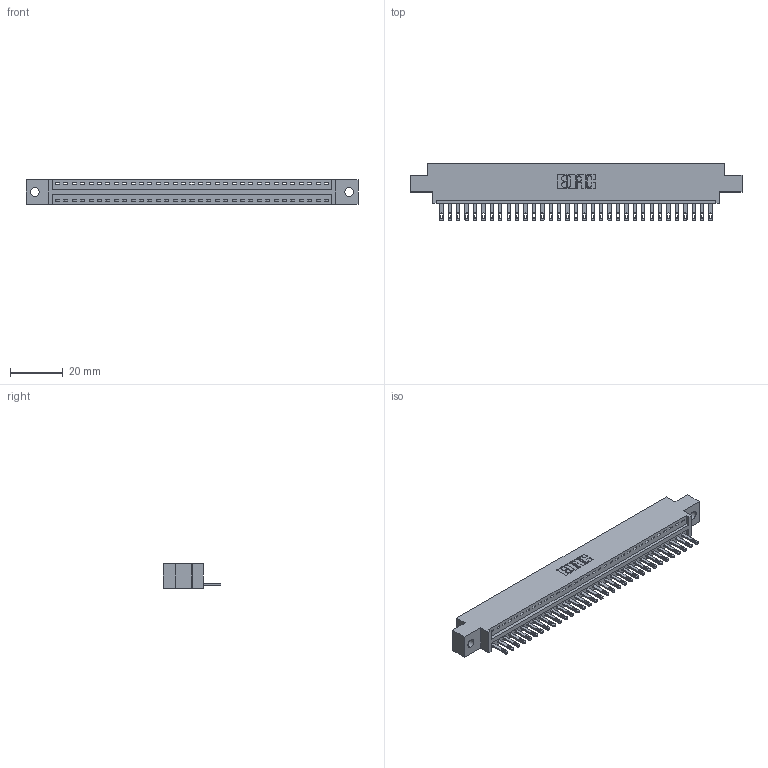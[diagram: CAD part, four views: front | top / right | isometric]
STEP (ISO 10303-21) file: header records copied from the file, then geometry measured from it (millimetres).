
FILE_DESCRIPTION (( 'STEP AP203' ), '1' );
FILE_NAME ('896-033-500-602.STEP', '2021-07-27T19:31:33', ( '' ), ( '' ), 'SwSTEP 2.0', 'SolidWorks 2020', '' );
FILE_SCHEMA (( 'CONFIG_CONTROL_DESIGN' ));
Length unit declared in the file: inch
Products named in the file (3): 896-033-500-602; 345-292-001_345-293-100; 846 Part_0.170 Offset - 0.128 Dia
Assembly tree (34 placements, depth 2):
  896-033-500-602
    846 Part_0.170 Offset - 0.128 Dia
    345-292-001_345-293-100  x33
Bounding box: 125.35 x 21.84 x 9.4 mm (x, y, z)
Volume: 11765.8 mm3; surface area: 14574.6 mm2
Topology: 34 solids, 34 shells, 1908 faces, 5885 edges, 3922 vertices
Faces by surface type: plane 1202, cylinder 706
Entity records: 21757 total; most frequent: CARTESIAN_POINT 3739, ORIENTED_EDGE 3706, DIRECTION 3311, EDGE_CURVE 1853, VECTOR 1585, LINE 1585, VERTEX_POINT 1234, AXIS2_PLACEMENT_3D 863
